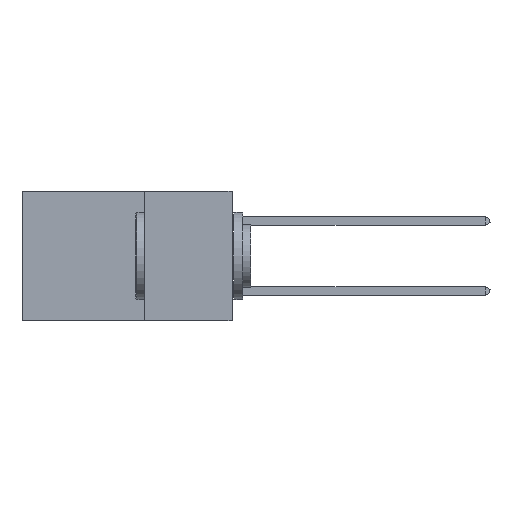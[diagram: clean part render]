
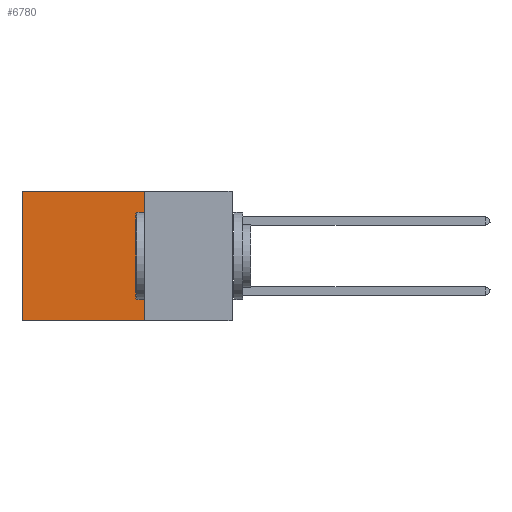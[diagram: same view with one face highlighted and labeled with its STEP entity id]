
A CAD part, left-side view. The second image highlights one B-rep face of the part: STEP entity #6780.
In plain terms, the highlighted planar face has unit normal (-1, 0, 0).
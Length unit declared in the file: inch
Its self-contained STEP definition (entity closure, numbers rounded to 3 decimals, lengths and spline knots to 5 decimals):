
#172 = VECTOR ( 'NONE', #15864, 39.37008 ) ;
#578 = FACE_OUTER_BOUND ( 'NONE', #3605, .T. ) ;
#833 = ORIENTED_EDGE ( 'NONE', *, *, #17018, .F. ) ;
#1040 = LINE ( 'NONE', #6210, #10661 ) ;
#1275 = DIRECTION ( 'NONE',  ( 1., 0., 0. ) ) ;
#2236 = ORIENTED_EDGE ( 'NONE', *, *, #22925, .F. ) ;
#3094 = CARTESIAN_POINT ( 'NONE',  ( 0.2875, 0.6, -0.37 ) ) ;
#3605 = EDGE_LOOP ( 'NONE', ( #16093, #833, #2236, #6378 ) ) ;
#4191 = LINE ( 'NONE', #16539, #21037 ) ;
#5112 = CARTESIAN_POINT ( 'NONE',  ( 0.2875, 0.25, -0.37 ) ) ;
#5825 = DIRECTION ( 'NONE',  ( 0., 0., -1. ) ) ;
#6210 = CARTESIAN_POINT ( 'NONE',  ( 0.2875, 0.25, 0. ) ) ;
#6378 = ORIENTED_EDGE ( 'NONE', *, *, #8513, .T. ) ;
#6780 = ADVANCED_FACE ( 'NONE', ( #578 ), #20884, .F. ) ;
#7008 = VERTEX_POINT ( 'NONE', #17991 ) ;
#7663 = VERTEX_POINT ( 'NONE', #3094 ) ;
#8048 = DIRECTION ( 'NONE',  ( 0., 0., -1. ) ) ;
#8513 = EDGE_CURVE ( 'NONE', #19202, #7008, #21217, .T. ) ;
#9263 = LINE ( 'NONE', #5112, #172 ) ;
#9600 = VECTOR ( 'NONE', #16017, 39.37008 ) ;
#10661 = VECTOR ( 'NONE', #8048, 39.37008 ) ;
#13044 = AXIS2_PLACEMENT_3D ( 'NONE', #22608, #1275, #13916 ) ;
#13916 = DIRECTION ( 'NONE',  ( 0., 0., -1. ) ) ;
#15864 = DIRECTION ( 'NONE',  ( 0., 1., 0. ) ) ;
#15889 = EDGE_CURVE ( 'NONE', #7008, #7663, #4191, .T. ) ;
#16017 = DIRECTION ( 'NONE',  ( 0., 1., 0. ) ) ;
#16093 = ORIENTED_EDGE ( 'NONE', *, *, #15889, .T. ) ;
#16539 = CARTESIAN_POINT ( 'NONE',  ( 0.2875, 0.6, 0. ) ) ;
#17018 = EDGE_CURVE ( 'NONE', #19815, #7663, #9263, .T. ) ;
#17991 = CARTESIAN_POINT ( 'NONE',  ( 0.2875, 0.6, 0. ) ) ;
#19202 = VERTEX_POINT ( 'NONE', #20140 ) ;
#19815 = VERTEX_POINT ( 'NONE', #23008 ) ;
#20140 = CARTESIAN_POINT ( 'NONE',  ( 0.2875, 0.25, 0. ) ) ;
#20884 = PLANE ( 'NONE',  #13044 ) ;
#21037 = VECTOR ( 'NONE', #5825, 39.37008 ) ;
#21217 = LINE ( 'NONE', #22986, #9600 ) ;
#22608 = CARTESIAN_POINT ( 'NONE',  ( 0.2875, 0.25, 0. ) ) ;
#22925 = EDGE_CURVE ( 'NONE', #19202, #19815, #1040, .T. ) ;
#22986 = CARTESIAN_POINT ( 'NONE',  ( 0.2875, 0.25, 0. ) ) ;
#23008 = CARTESIAN_POINT ( 'NONE',  ( 0.2875, 0.25, -0.37 ) ) ;
